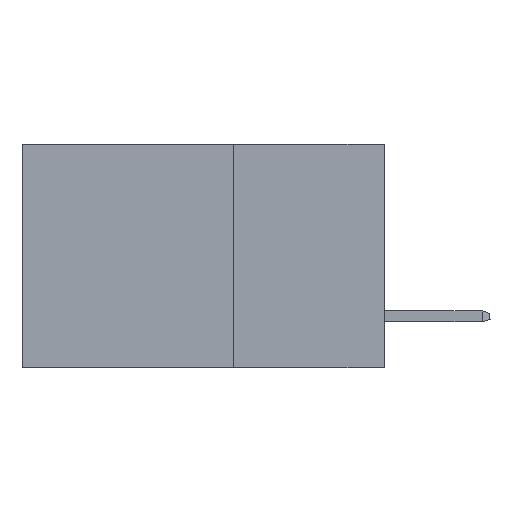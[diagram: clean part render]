
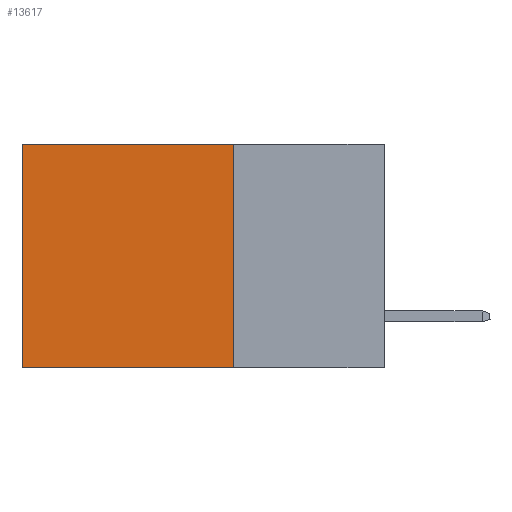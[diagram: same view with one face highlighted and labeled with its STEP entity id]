
A CAD part, left-side view. The second image highlights one B-rep face of the part: STEP entity #13617.
In plain terms, the highlighted planar face has unit normal (-1, 0, 0).
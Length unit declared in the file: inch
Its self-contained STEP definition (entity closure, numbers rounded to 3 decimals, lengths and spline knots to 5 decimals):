
#593 = VECTOR ( 'NONE', #21246, 39.37008 ) ;
#2781 = CARTESIAN_POINT ( 'NONE',  ( 0.298, 0.6, 0. ) ) ;
#3384 = CARTESIAN_POINT ( 'NONE',  ( 0.298, 0.25, -0.37 ) ) ;
#5465 = DIRECTION ( 'NONE',  ( 1., 0., 0. ) ) ;
#6123 = CARTESIAN_POINT ( 'NONE',  ( 0.298, 0.25, 0. ) ) ;
#6291 = VECTOR ( 'NONE', #10730, 39.37008 ) ;
#9209 = EDGE_LOOP ( 'NONE', ( #10501, #31534, #16527, #19321 ) ) ;
#10460 = DIRECTION ( 'NONE',  ( 0., 0., -1. ) ) ;
#10501 = ORIENTED_EDGE ( 'NONE', *, *, #14668, .T. ) ;
#10730 = DIRECTION ( 'NONE',  ( 0., 1., 0. ) ) ;
#13617 = ADVANCED_FACE ( 'NONE', ( #30359 ), #18205, .F. ) ;
#14668 = EDGE_CURVE ( 'NONE', #32446, #26358, #25457, .T. ) ;
#16527 = ORIENTED_EDGE ( 'NONE', *, *, #18108, .F. ) ;
#16991 = VERTEX_POINT ( 'NONE', #25677 ) ;
#17791 = LINE ( 'NONE', #6123, #593 ) ;
#18108 = EDGE_CURVE ( 'NONE', #16991, #22607, #17791, .T. ) ;
#18205 = PLANE ( 'NONE',  #28575 ) ;
#18352 = CARTESIAN_POINT ( 'NONE',  ( 0.298, 0.25, 0. ) ) ;
#18488 = DIRECTION ( 'NONE',  ( 0., 1., 0. ) ) ;
#19321 = ORIENTED_EDGE ( 'NONE', *, *, #27700, .T. ) ;
#20808 = CARTESIAN_POINT ( 'NONE',  ( 0.298, 0.25, 0. ) ) ;
#21246 = DIRECTION ( 'NONE',  ( 0., 0., -1. ) ) ;
#22297 = VECTOR ( 'NONE', #10460, 39.37008 ) ;
#22607 = VERTEX_POINT ( 'NONE', #25302 ) ;
#23343 = DIRECTION ( 'NONE',  ( 0., 0., -1. ) ) ;
#25302 = CARTESIAN_POINT ( 'NONE',  ( 0.298, 0.25, -0.37 ) ) ;
#25457 = LINE ( 'NONE', #2781, #22297 ) ;
#25677 = CARTESIAN_POINT ( 'NONE',  ( 0.298, 0.25, 0. ) ) ;
#26358 = VERTEX_POINT ( 'NONE', #30439 ) ;
#27207 = EDGE_CURVE ( 'NONE', #22607, #26358, #29507, .T. ) ;
#27700 = EDGE_CURVE ( 'NONE', #16991, #32446, #30639, .T. ) ;
#28308 = VECTOR ( 'NONE', #18488, 39.37008 ) ;
#28575 = AXIS2_PLACEMENT_3D ( 'NONE', #20808, #5465, #23343 ) ;
#29507 = LINE ( 'NONE', #3384, #28308 ) ;
#30359 = FACE_OUTER_BOUND ( 'NONE', #9209, .T. ) ;
#30439 = CARTESIAN_POINT ( 'NONE',  ( 0.298, 0.6, -0.37 ) ) ;
#30639 = LINE ( 'NONE', #18352, #6291 ) ;
#30806 = CARTESIAN_POINT ( 'NONE',  ( 0.298, 0.6, 0. ) ) ;
#31534 = ORIENTED_EDGE ( 'NONE', *, *, #27207, .F. ) ;
#32446 = VERTEX_POINT ( 'NONE', #30806 ) ;
